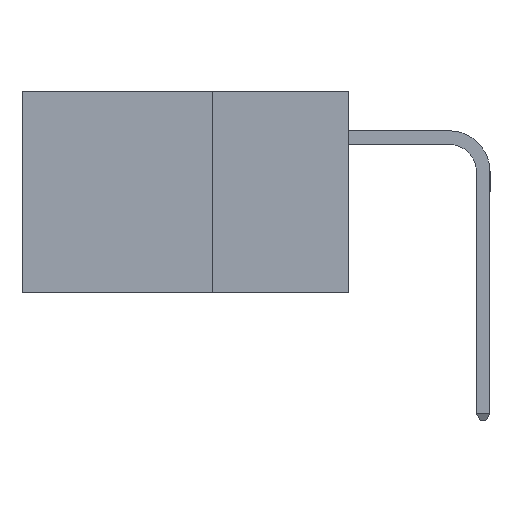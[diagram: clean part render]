
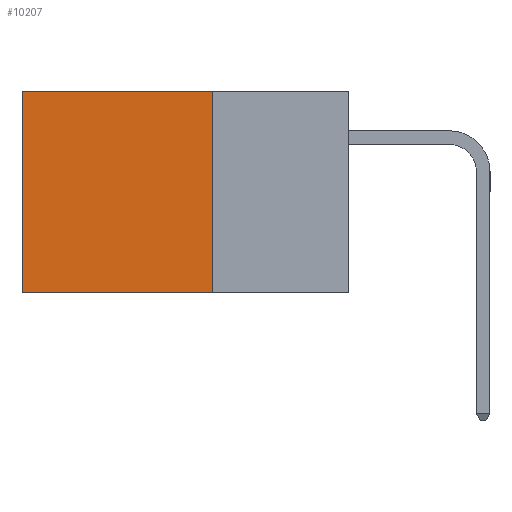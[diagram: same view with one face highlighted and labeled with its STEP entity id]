
A CAD part, left-side view. The second image highlights one B-rep face of the part: STEP entity #10207.
In plain terms, the highlighted planar face has unit normal (-1, 0, 0).
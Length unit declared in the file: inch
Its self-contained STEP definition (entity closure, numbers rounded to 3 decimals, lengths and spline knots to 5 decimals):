
#298 = DIRECTION ( 'NONE',  ( 0., 0., -1. ) ) ;
#509 = EDGE_LOOP ( 'NONE', ( #10842, #1951, #9937, #8104 ) ) ;
#531 = LINE ( 'NONE', #4323, #5650 ) ;
#1788 = VERTEX_POINT ( 'NONE', #7468 ) ;
#1917 = VECTOR ( 'NONE', #298, 39.37008 ) ;
#1951 = ORIENTED_EDGE ( 'NONE', *, *, #9233, .F. ) ;
#2076 = CARTESIAN_POINT ( 'NONE',  ( 0.2875, 0.25, -0.37 ) ) ;
#2161 = VERTEX_POINT ( 'NONE', #6060 ) ;
#4156 = DIRECTION ( 'NONE',  ( 0., 1., 0. ) ) ;
#4309 = VECTOR ( 'NONE', #4156, 39.37008 ) ;
#4323 = CARTESIAN_POINT ( 'NONE',  ( 0.2875, 0.25, 0. ) ) ;
#4505 = LINE ( 'NONE', #6905, #1917 ) ;
#4731 = PLANE ( 'NONE',  #6259 ) ;
#5307 = FACE_OUTER_BOUND ( 'NONE', #509, .T. ) ;
#5567 = VERTEX_POINT ( 'NONE', #2076 ) ;
#5650 = VECTOR ( 'NONE', #10623, 39.37008 ) ;
#5691 = CARTESIAN_POINT ( 'NONE',  ( 0.2875, 0.25, 0. ) ) ;
#6060 = CARTESIAN_POINT ( 'NONE',  ( 0.2875, 0.6, 0. ) ) ;
#6259 = AXIS2_PLACEMENT_3D ( 'NONE', #5691, #11884, #6621 ) ;
#6621 = DIRECTION ( 'NONE',  ( 0., 0., -1. ) ) ;
#6905 = CARTESIAN_POINT ( 'NONE',  ( 0.2875, 0.6, 0. ) ) ;
#7468 = CARTESIAN_POINT ( 'NONE',  ( 0.2875, 0.6, -0.37 ) ) ;
#7524 = CARTESIAN_POINT ( 'NONE',  ( 0.2875, 0.25, 0. ) ) ;
#7731 = EDGE_CURVE ( 'NONE', #9463, #5567, #11393, .T. ) ;
#7805 = CARTESIAN_POINT ( 'NONE',  ( 0.2875, 0.25, -0.37 ) ) ;
#8078 = EDGE_CURVE ( 'NONE', #9463, #2161, #531, .T. ) ;
#8104 = ORIENTED_EDGE ( 'NONE', *, *, #8078, .T. ) ;
#8119 = CARTESIAN_POINT ( 'NONE',  ( 0.2875, 0.25, 0. ) ) ;
#9045 = VECTOR ( 'NONE', #10180, 39.37008 ) ;
#9233 = EDGE_CURVE ( 'NONE', #5567, #1788, #11488, .T. ) ;
#9463 = VERTEX_POINT ( 'NONE', #8119 ) ;
#9937 = ORIENTED_EDGE ( 'NONE', *, *, #7731, .F. ) ;
#10180 = DIRECTION ( 'NONE',  ( 0., 0., -1. ) ) ;
#10207 = ADVANCED_FACE ( 'NONE', ( #5307 ), #4731, .F. ) ;
#10447 = EDGE_CURVE ( 'NONE', #2161, #1788, #4505, .T. ) ;
#10623 = DIRECTION ( 'NONE',  ( 0., 1., 0. ) ) ;
#10842 = ORIENTED_EDGE ( 'NONE', *, *, #10447, .T. ) ;
#11393 = LINE ( 'NONE', #7524, #9045 ) ;
#11488 = LINE ( 'NONE', #7805, #4309 ) ;
#11884 = DIRECTION ( 'NONE',  ( 1., 0., 0. ) ) ;
